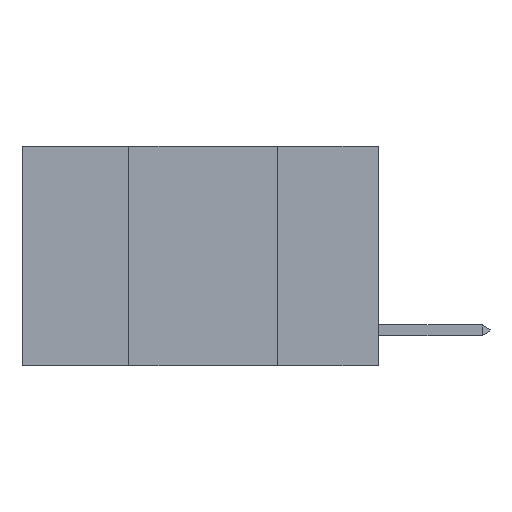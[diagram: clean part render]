
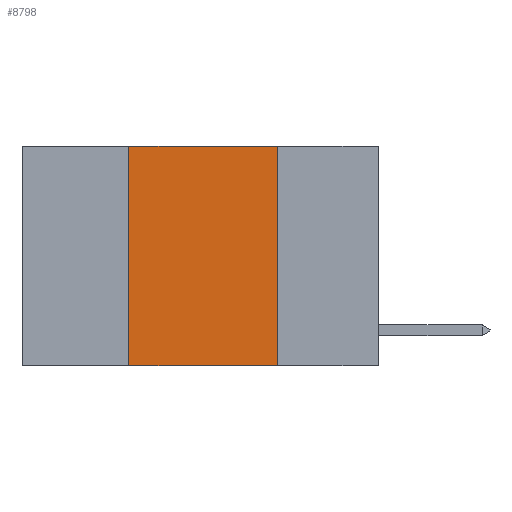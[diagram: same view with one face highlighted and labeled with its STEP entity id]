
A CAD part, left-side view. The second image highlights one B-rep face of the part: STEP entity #8798.
In plain terms, the highlighted planar face has unit normal (-1, 0, 0).
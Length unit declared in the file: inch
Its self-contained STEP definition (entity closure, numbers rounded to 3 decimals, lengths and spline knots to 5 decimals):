
#133 = VERTEX_POINT ( 'NONE', #8392 ) ;
#517 = EDGE_CURVE ( 'NONE', #9710, #133, #5157, .T. ) ;
#1243 = VECTOR ( 'NONE', #11658, 39.37008 ) ;
#2106 = CARTESIAN_POINT ( 'NONE',  ( 0., 0.17, 0. ) ) ;
#2573 = CARTESIAN_POINT ( 'NONE',  ( 0., 0.42, -0.37 ) ) ;
#2838 = DIRECTION ( 'NONE',  ( 1., 0., 0. ) ) ;
#2863 = EDGE_LOOP ( 'NONE', ( #7672, #11817, #2948, #10589 ) ) ;
#2948 = ORIENTED_EDGE ( 'NONE', *, *, #7632, .F. ) ;
#3065 = VECTOR ( 'NONE', #9071, 39.37008 ) ;
#3122 = EDGE_CURVE ( 'NONE', #8549, #6798, #5098, .T. ) ;
#3555 = DIRECTION ( 'NONE',  ( 0., 0., 1. ) ) ;
#3812 = LINE ( 'NONE', #7508, #5691 ) ;
#4769 = EDGE_CURVE ( 'NONE', #6798, #133, #3812, .T. ) ;
#5098 = LINE ( 'NONE', #7016, #1243 ) ;
#5157 = LINE ( 'NONE', #11085, #3065 ) ;
#5661 = DIRECTION ( 'NONE',  ( 0., 0., -1. ) ) ;
#5691 = VECTOR ( 'NONE', #5661, 39.37008 ) ;
#6328 = AXIS2_PLACEMENT_3D ( 'NONE', #12408, #2838, #9613 ) ;
#6673 = CARTESIAN_POINT ( 'NONE',  ( 0., 0.42, 0. ) ) ;
#6798 = VERTEX_POINT ( 'NONE', #2106 ) ;
#7016 = CARTESIAN_POINT ( 'NONE',  ( 0., 0.6, 0. ) ) ;
#7508 = CARTESIAN_POINT ( 'NONE',  ( 0., 0.17, 0. ) ) ;
#7564 = PLANE ( 'NONE',  #6328 ) ;
#7632 = EDGE_CURVE ( 'NONE', #9710, #8549, #12530, .T. ) ;
#7672 = ORIENTED_EDGE ( 'NONE', *, *, #4769, .F. ) ;
#8392 = CARTESIAN_POINT ( 'NONE',  ( 0., 0.17, -0.37 ) ) ;
#8549 = VERTEX_POINT ( 'NONE', #11712 ) ;
#8798 = ADVANCED_FACE ( 'NONE', ( #12533 ), #7564, .F. ) ;
#9071 = DIRECTION ( 'NONE',  ( 0., -1., 0. ) ) ;
#9613 = DIRECTION ( 'NONE',  ( 0., 0., -1. ) ) ;
#9710 = VERTEX_POINT ( 'NONE', #2573 ) ;
#10589 = ORIENTED_EDGE ( 'NONE', *, *, #517, .T. ) ;
#11085 = CARTESIAN_POINT ( 'NONE',  ( 0., 0.6, -0.37 ) ) ;
#11658 = DIRECTION ( 'NONE',  ( 0., -1., 0. ) ) ;
#11712 = CARTESIAN_POINT ( 'NONE',  ( 0., 0.42, 0. ) ) ;
#11817 = ORIENTED_EDGE ( 'NONE', *, *, #3122, .F. ) ;
#11977 = VECTOR ( 'NONE', #3555, 39.37008 ) ;
#12408 = CARTESIAN_POINT ( 'NONE',  ( 0., 0.6, 0. ) ) ;
#12530 = LINE ( 'NONE', #6673, #11977 ) ;
#12533 = FACE_OUTER_BOUND ( 'NONE', #2863, .T. ) ;
